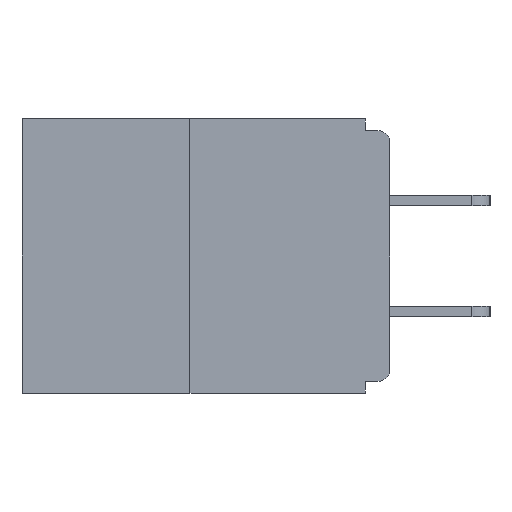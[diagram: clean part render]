
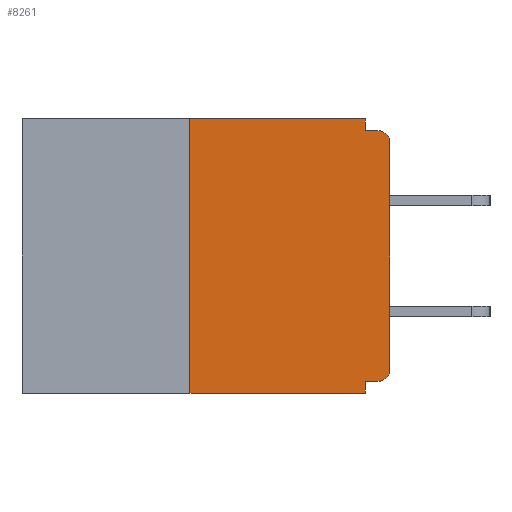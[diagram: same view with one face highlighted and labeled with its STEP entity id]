
A CAD part, left-side view. The second image highlights one B-rep face of the part: STEP entity #8261.
In plain terms, the highlighted planar face has unit normal (-1, 0, 0).
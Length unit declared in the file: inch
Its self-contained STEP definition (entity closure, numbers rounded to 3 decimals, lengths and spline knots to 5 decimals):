
#141 = CARTESIAN_POINT ( 'NONE',  ( 0., 0.015, -0.03 ) ) ;
#287 = DIRECTION ( 'NONE',  ( 0., 0., -1. ) ) ;
#437 = DIRECTION ( 'NONE',  ( 0., -1., 0. ) ) ;
#462 = DIRECTION ( 'NONE',  ( -1., 0., 0. ) ) ;
#633 = EDGE_CURVE ( 'NONE', #1830, #4603, #6387, .T. ) ;
#651 = EDGE_LOOP ( 'NONE', ( #7561, #1772, #2609, #918, #10656, #7627, #1306, #2058, #4210, #4785 ) ) ;
#891 = CARTESIAN_POINT ( 'NONE',  ( 0., 0.46, -0.343 ) ) ;
#918 = ORIENTED_EDGE ( 'NONE', *, *, #633, .F. ) ;
#997 = DIRECTION ( 'NONE',  ( 0., -1., 0. ) ) ;
#1050 = EDGE_CURVE ( 'NONE', #6420, #5756, #4324, .T. ) ;
#1306 = ORIENTED_EDGE ( 'NONE', *, *, #9822, .T. ) ;
#1772 = ORIENTED_EDGE ( 'NONE', *, *, #8513, .F. ) ;
#1775 = DIRECTION ( 'NONE',  ( -1., 0., 0. ) ) ;
#1783 = CARTESIAN_POINT ( 'NONE',  ( 0., 0.031, -0.328 ) ) ;
#1801 = DIRECTION ( 'NONE',  ( 1., 0., 0. ) ) ;
#1830 = VERTEX_POINT ( 'NONE', #1783 ) ;
#1906 = CARTESIAN_POINT ( 'NONE',  ( 0., 0., 0. ) ) ;
#1937 = CARTESIAN_POINT ( 'NONE',  ( 0., 0.031, 0. ) ) ;
#2041 = LINE ( 'NONE', #5451, #8562 ) ;
#2058 = ORIENTED_EDGE ( 'NONE', *, *, #1050, .T. ) ;
#2609 = ORIENTED_EDGE ( 'NONE', *, *, #11154, .T. ) ;
#2696 = FACE_OUTER_BOUND ( 'NONE', #651, .T. ) ;
#3075 = DIRECTION ( 'NONE',  ( 0., 0., -1. ) ) ;
#3184 = EDGE_CURVE ( 'NONE', #4659, #5756, #3977, .T. ) ;
#3226 = VECTOR ( 'NONE', #3381, 39.37008 ) ;
#3356 = VECTOR ( 'NONE', #7213, 39.37008 ) ;
#3381 = DIRECTION ( 'NONE',  ( 0., 0., 1. ) ) ;
#3522 = CARTESIAN_POINT ( 'NONE',  ( 0., 0.015, -0.328 ) ) ;
#3624 = DIRECTION ( 'NONE',  ( 0., 0., -1. ) ) ;
#3904 = CARTESIAN_POINT ( 'NONE',  ( 0., 0.031, -0.343 ) ) ;
#3977 = LINE ( 'NONE', #10064, #5516 ) ;
#4046 = EDGE_CURVE ( 'NONE', #9061, #7979, #6734, .T. ) ;
#4125 = EDGE_CURVE ( 'NONE', #9061, #1830, #2041, .T. ) ;
#4210 = ORIENTED_EDGE ( 'NONE', *, *, #3184, .F. ) ;
#4324 = CIRCLE ( 'NONE', #6683, 0.015 ) ;
#4382 = LINE ( 'NONE', #8072, #3356 ) ;
#4603 = VERTEX_POINT ( 'NONE', #4746 ) ;
#4659 = VERTEX_POINT ( 'NONE', #8172 ) ;
#4746 = CARTESIAN_POINT ( 'NONE',  ( 0., 0.031, -0.343 ) ) ;
#4785 = ORIENTED_EDGE ( 'NONE', *, *, #9551, .F. ) ;
#4929 = AXIS2_PLACEMENT_3D ( 'NONE', #8152, #462, #287 ) ;
#5022 = CARTESIAN_POINT ( 'NONE',  ( 0., 0.015, -0.015 ) ) ;
#5061 = LINE ( 'NONE', #9513, #3226 ) ;
#5275 = DIRECTION ( 'NONE',  ( 0., 0., 1. ) ) ;
#5341 = AXIS2_PLACEMENT_3D ( 'NONE', #6076, #1801, #8764 ) ;
#5451 = CARTESIAN_POINT ( 'NONE',  ( 0., 0., -0.328 ) ) ;
#5516 = VECTOR ( 'NONE', #437, 39.37008 ) ;
#5617 = VECTOR ( 'NONE', #3624, 39.37008 ) ;
#5756 = VERTEX_POINT ( 'NONE', #5022 ) ;
#5841 = CARTESIAN_POINT ( 'NONE',  ( 0., 0.25, -0.343 ) ) ;
#5869 = VERTEX_POINT ( 'NONE', #9807 ) ;
#6033 = VECTOR ( 'NONE', #5275, 39.37008 ) ;
#6076 = CARTESIAN_POINT ( 'NONE',  ( 0., 0.46, 0. ) ) ;
#6270 = LINE ( 'NONE', #1937, #5617 ) ;
#6387 = LINE ( 'NONE', #3904, #7434 ) ;
#6420 = VERTEX_POINT ( 'NONE', #8900 ) ;
#6683 = AXIS2_PLACEMENT_3D ( 'NONE', #141, #1775, #9526 ) ;
#6734 = CIRCLE ( 'NONE', #4929, 0.015 ) ;
#7213 = DIRECTION ( 'NONE',  ( 0., -1., 0. ) ) ;
#7434 = VECTOR ( 'NONE', #3075, 39.37008 ) ;
#7561 = ORIENTED_EDGE ( 'NONE', *, *, #8625, .F. ) ;
#7627 = ORIENTED_EDGE ( 'NONE', *, *, #4046, .T. ) ;
#7979 = VERTEX_POINT ( 'NONE', #11063 ) ;
#8072 = CARTESIAN_POINT ( 'NONE',  ( 0., 0.46, 0. ) ) ;
#8152 = CARTESIAN_POINT ( 'NONE',  ( 0., 0.015, -0.313 ) ) ;
#8172 = CARTESIAN_POINT ( 'NONE',  ( 0., 0.031, -0.015 ) ) ;
#8261 = ADVANCED_FACE ( 'NONE', ( #2696 ), #10529, .F. ) ;
#8499 = LINE ( 'NONE', #1906, #6033 ) ;
#8513 = EDGE_CURVE ( 'NONE', #11077, #5869, #5061, .T. ) ;
#8562 = VECTOR ( 'NONE', #9856, 39.37008 ) ;
#8625 = EDGE_CURVE ( 'NONE', #5869, #10302, #4382, .T. ) ;
#8763 = LINE ( 'NONE', #891, #10606 ) ;
#8764 = DIRECTION ( 'NONE',  ( 0., 0., -1. ) ) ;
#8900 = CARTESIAN_POINT ( 'NONE',  ( 0., 0., -0.03 ) ) ;
#9061 = VERTEX_POINT ( 'NONE', #3522 ) ;
#9495 = CARTESIAN_POINT ( 'NONE',  ( 0., 0.031, 0. ) ) ;
#9513 = CARTESIAN_POINT ( 'NONE',  ( 0., 0.25, 0. ) ) ;
#9526 = DIRECTION ( 'NONE',  ( 0., 0., -1. ) ) ;
#9551 = EDGE_CURVE ( 'NONE', #10302, #4659, #6270, .T. ) ;
#9807 = CARTESIAN_POINT ( 'NONE',  ( 0., 0.25, 0. ) ) ;
#9822 = EDGE_CURVE ( 'NONE', #7979, #6420, #8499, .T. ) ;
#9856 = DIRECTION ( 'NONE',  ( 0., 1., 0. ) ) ;
#10064 = CARTESIAN_POINT ( 'NONE',  ( 0., 0., -0.015 ) ) ;
#10302 = VERTEX_POINT ( 'NONE', #9495 ) ;
#10529 = PLANE ( 'NONE',  #5341 ) ;
#10606 = VECTOR ( 'NONE', #997, 39.37008 ) ;
#10656 = ORIENTED_EDGE ( 'NONE', *, *, #4125, .F. ) ;
#11063 = CARTESIAN_POINT ( 'NONE',  ( 0., 0., -0.313 ) ) ;
#11077 = VERTEX_POINT ( 'NONE', #5841 ) ;
#11154 = EDGE_CURVE ( 'NONE', #11077, #4603, #8763, .T. ) ;
